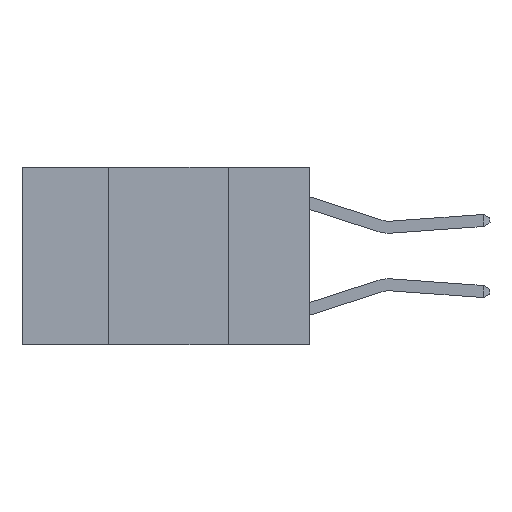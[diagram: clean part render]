
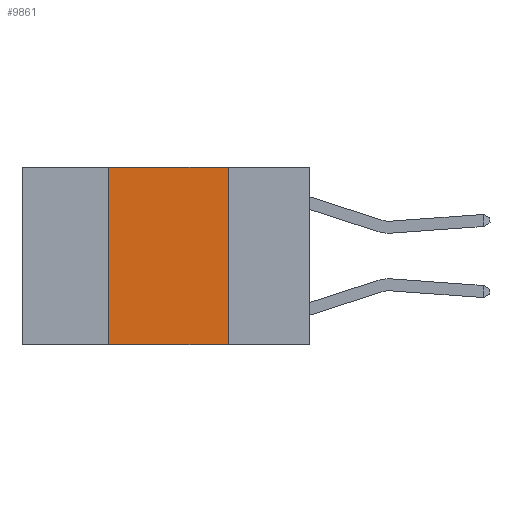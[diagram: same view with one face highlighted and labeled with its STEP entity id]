
A CAD part, left-side view. The second image highlights one B-rep face of the part: STEP entity #9861.
In plain terms, the highlighted planar face has unit normal (-1, 0, 0).
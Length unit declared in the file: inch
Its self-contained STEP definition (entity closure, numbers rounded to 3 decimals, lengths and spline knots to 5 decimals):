
#1264 = EDGE_CURVE ( 'NONE', #27353, #3734, #13096, .T. ) ;
#1299 = DIRECTION ( 'NONE',  ( 0., 0., -1. ) ) ;
#2391 = CARTESIAN_POINT ( 'NONE',  ( 0., 0.42, 0. ) ) ;
#3395 = EDGE_CURVE ( 'NONE', #3734, #13389, #11115, .T. ) ;
#3734 = VERTEX_POINT ( 'NONE', #7429 ) ;
#4116 = VECTOR ( 'NONE', #18354, 39.37008 ) ;
#4249 = CARTESIAN_POINT ( 'NONE',  ( 0., 0.6, -0.37 ) ) ;
#5646 = FACE_OUTER_BOUND ( 'NONE', #19902, .T. ) ;
#6015 = ORIENTED_EDGE ( 'NONE', *, *, #3395, .F. ) ;
#6850 = VECTOR ( 'NONE', #22131, 39.37008 ) ;
#7429 = CARTESIAN_POINT ( 'NONE',  ( 0., 0.17, 0. ) ) ;
#9373 = LINE ( 'NONE', #11998, #14905 ) ;
#9861 = ADVANCED_FACE ( 'NONE', ( #5646 ), #11594, .F. ) ;
#11115 = LINE ( 'NONE', #15543, #24204 ) ;
#11403 = CARTESIAN_POINT ( 'NONE',  ( 0., 0.17, -0.37 ) ) ;
#11594 = PLANE ( 'NONE',  #22293 ) ;
#11998 = CARTESIAN_POINT ( 'NONE',  ( 0., 0.42, 0. ) ) ;
#12994 = ORIENTED_EDGE ( 'NONE', *, *, #1264, .F. ) ;
#13096 = LINE ( 'NONE', #15129, #6850 ) ;
#13389 = VERTEX_POINT ( 'NONE', #11403 ) ;
#13960 = DIRECTION ( 'NONE',  ( 0., 0., -1. ) ) ;
#14905 = VECTOR ( 'NONE', #16635, 39.37008 ) ;
#15129 = CARTESIAN_POINT ( 'NONE',  ( 0., 0.6, 0. ) ) ;
#15543 = CARTESIAN_POINT ( 'NONE',  ( 0., 0.17, 0. ) ) ;
#15574 = VERTEX_POINT ( 'NONE', #19087 ) ;
#16635 = DIRECTION ( 'NONE',  ( 0., 0., 1. ) ) ;
#16658 = LINE ( 'NONE', #4249, #4116 ) ;
#18354 = DIRECTION ( 'NONE',  ( 0., -1., 0. ) ) ;
#19087 = CARTESIAN_POINT ( 'NONE',  ( 0., 0.42, -0.37 ) ) ;
#19902 = EDGE_LOOP ( 'NONE', ( #6015, #12994, #25330, #26026 ) ) ;
#21275 = EDGE_CURVE ( 'NONE', #15574, #13389, #16658, .T. ) ;
#22131 = DIRECTION ( 'NONE',  ( 0., -1., 0. ) ) ;
#22293 = AXIS2_PLACEMENT_3D ( 'NONE', #25480, #27792, #13960 ) ;
#24204 = VECTOR ( 'NONE', #1299, 39.37008 ) ;
#25330 = ORIENTED_EDGE ( 'NONE', *, *, #28971, .F. ) ;
#25480 = CARTESIAN_POINT ( 'NONE',  ( 0., 0.6, 0. ) ) ;
#26026 = ORIENTED_EDGE ( 'NONE', *, *, #21275, .T. ) ;
#27353 = VERTEX_POINT ( 'NONE', #2391 ) ;
#27792 = DIRECTION ( 'NONE',  ( 1., 0., 0. ) ) ;
#28971 = EDGE_CURVE ( 'NONE', #15574, #27353, #9373, .T. ) ;
